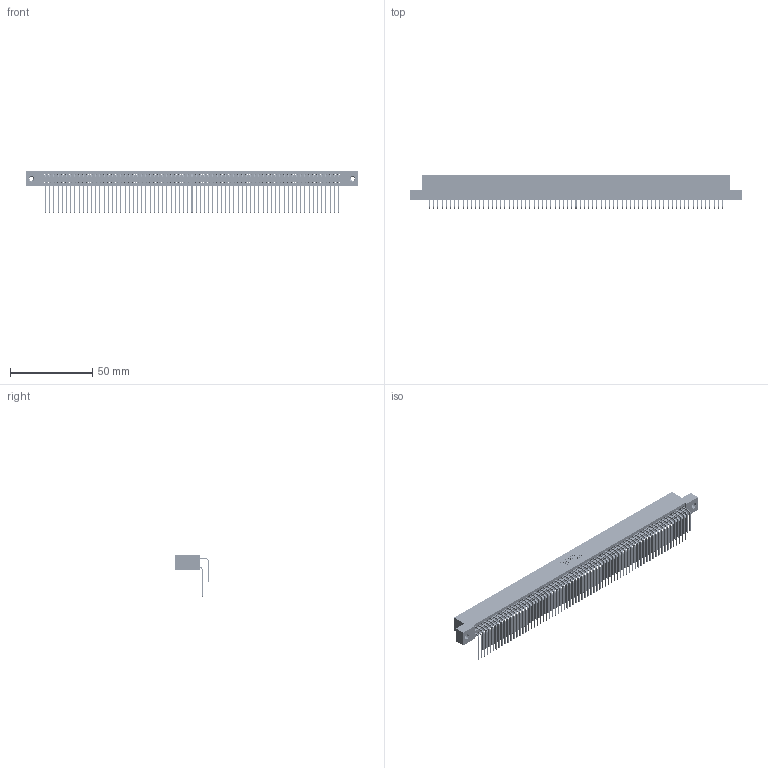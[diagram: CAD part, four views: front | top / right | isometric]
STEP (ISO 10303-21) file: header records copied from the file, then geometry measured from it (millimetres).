
FILE_DESCRIPTION (( 'STEP AP203' ), '1' );
FILE_NAME ('395-142-559-207.STEP', '2018-12-06T04:59:22', ( '' ), ( '' ), 'SwSTEP 2.0', 'SolidWorks 2016', '' );
FILE_SCHEMA (( 'CONFIG_CONTROL_DESIGN' ));
Length unit declared in the file: inch
Products named in the file (5): 345 Part_Flush Mounting Lugs - 0.156 Dia-TI; 345-292-001_559 Tail - 2; 345-292-001_558 559 Tail - 1; 395-142-559-207; 345-250-001_345-250-005-103
Assembly tree (145 placements, depth 2):
  395-142-559-207
    345 Part_Flush Mounting Lugs - 0.156 Dia-TI
    345-292-001_558 559 Tail - 1  x71
    345-292-001_559 Tail - 2  x71
    345-250-001_345-250-005-103  x2
Bounding box: 201.55 x 20.56 x 25.53 mm (x, y, z)
Volume: 20653.5 mm3; surface area: 34970.9 mm2
Topology: 145 solids, 145 shells, 7570 faces, 22487 edges, 14794 vertices
Faces by surface type: plane 5082, cylinder 2472, cone 12, torus 4
Entity records: 54642 total; most frequent: CARTESIAN_POINT 9158, ORIENTED_EDGE 9034, DIRECTION 8039, EDGE_CURVE 4517, VECTOR 4041, LINE 4041, VERTEX_POINT 3004, AXIS2_PLACEMENT_3D 1999
